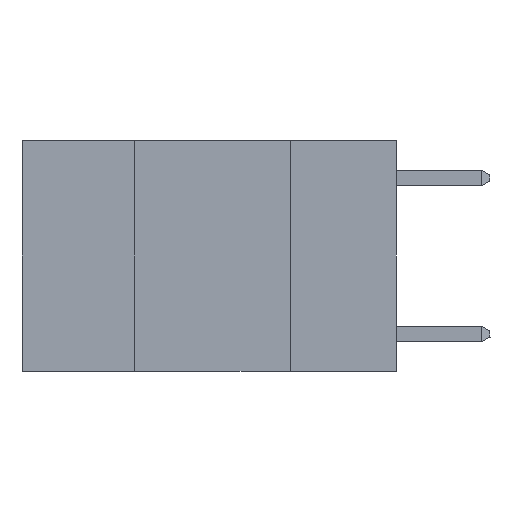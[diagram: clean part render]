
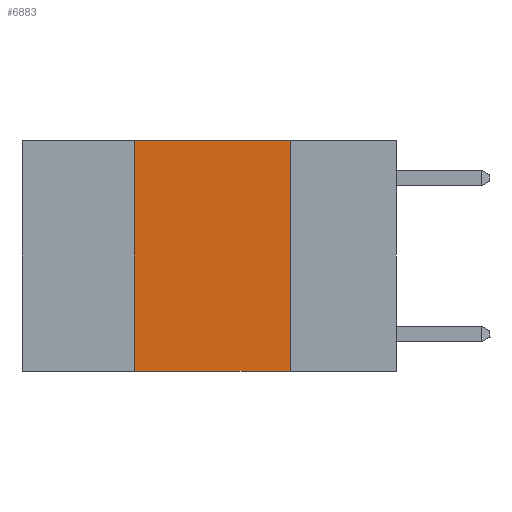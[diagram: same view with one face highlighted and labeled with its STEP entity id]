
A CAD part, left-side view. The second image highlights one B-rep face of the part: STEP entity #6883.
In plain terms, the highlighted planar face has unit normal (-1, 0, 0).
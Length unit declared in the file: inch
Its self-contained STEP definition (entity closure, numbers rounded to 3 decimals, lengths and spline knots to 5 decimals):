
#124 = ORIENTED_EDGE ( 'NONE', *, *, #10872, .F. ) ;
#139 = ORIENTED_EDGE ( 'NONE', *, *, #1727, .F. ) ;
#192 = ORIENTED_EDGE ( 'NONE', *, *, #11482, .F. ) ;
#214 = ORIENTED_EDGE ( 'NONE', *, *, #12075, .T. ) ;
#1079 = VERTEX_POINT ( 'NONE', #11744 ) ;
#1254 = LINE ( 'NONE', #6306, #9176 ) ;
#1347 = FACE_OUTER_BOUND ( 'NONE', #2479, .T. ) ;
#1727 = EDGE_CURVE ( 'NONE', #10796, #7311, #7254, .T. ) ;
#2259 = CARTESIAN_POINT ( 'NONE',  ( 0., 0.17, 0. ) ) ;
#2479 = EDGE_LOOP ( 'NONE', ( #124, #139, #192, #214 ) ) ;
#3089 = VECTOR ( 'NONE', #4526, 39.37008 ) ;
#3425 = LINE ( 'NONE', #11359, #3089 ) ;
#3862 = PLANE ( 'NONE',  #7108 ) ;
#3896 = DIRECTION ( 'NONE',  ( 0., 0., -1. ) ) ;
#3920 = DIRECTION ( 'NONE',  ( 0., -1., 0. ) ) ;
#4406 = CARTESIAN_POINT ( 'NONE',  ( 0., 0.6, 0. ) ) ;
#4526 = DIRECTION ( 'NONE',  ( 0., 0., 1. ) ) ;
#4997 = DIRECTION ( 'NONE',  ( 1., 0., 0. ) ) ;
#5142 = VECTOR ( 'NONE', #3896, 39.37008 ) ;
#6233 = VERTEX_POINT ( 'NONE', #12677 ) ;
#6306 = CARTESIAN_POINT ( 'NONE',  ( 0., 0.6, -0.37 ) ) ;
#6883 = ADVANCED_FACE ( 'NONE', ( #1347 ), #3862, .F. ) ;
#7108 = AXIS2_PLACEMENT_3D ( 'NONE', #8032, #4997, #11732 ) ;
#7254 = LINE ( 'NONE', #4406, #11618 ) ;
#7311 = VERTEX_POINT ( 'NONE', #2259 ) ;
#7328 = DIRECTION ( 'NONE',  ( 0., -1., 0. ) ) ;
#7861 = LINE ( 'NONE', #10815, #5142 ) ;
#8032 = CARTESIAN_POINT ( 'NONE',  ( 0., 0.6, 0. ) ) ;
#9176 = VECTOR ( 'NONE', #7328, 39.37008 ) ;
#10796 = VERTEX_POINT ( 'NONE', #11687 ) ;
#10815 = CARTESIAN_POINT ( 'NONE',  ( 0., 0.17, 0. ) ) ;
#10872 = EDGE_CURVE ( 'NONE', #7311, #6233, #7861, .T. ) ;
#11359 = CARTESIAN_POINT ( 'NONE',  ( 0., 0.42, 0. ) ) ;
#11482 = EDGE_CURVE ( 'NONE', #1079, #10796, #3425, .T. ) ;
#11618 = VECTOR ( 'NONE', #3920, 39.37008 ) ;
#11687 = CARTESIAN_POINT ( 'NONE',  ( 0., 0.42, 0. ) ) ;
#11732 = DIRECTION ( 'NONE',  ( 0., 0., -1. ) ) ;
#11744 = CARTESIAN_POINT ( 'NONE',  ( 0., 0.42, -0.37 ) ) ;
#12075 = EDGE_CURVE ( 'NONE', #1079, #6233, #1254, .T. ) ;
#12677 = CARTESIAN_POINT ( 'NONE',  ( 0., 0.17, -0.37 ) ) ;
